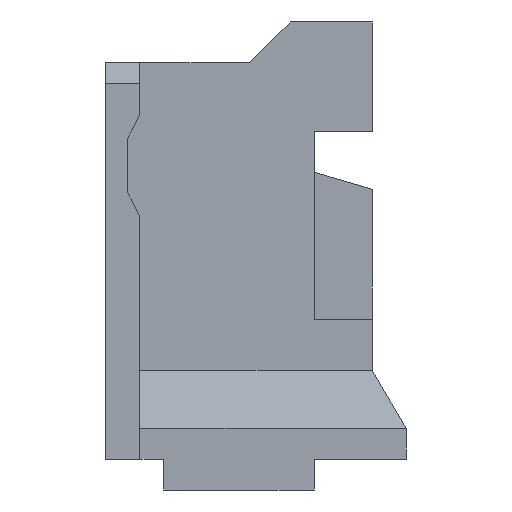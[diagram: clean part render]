
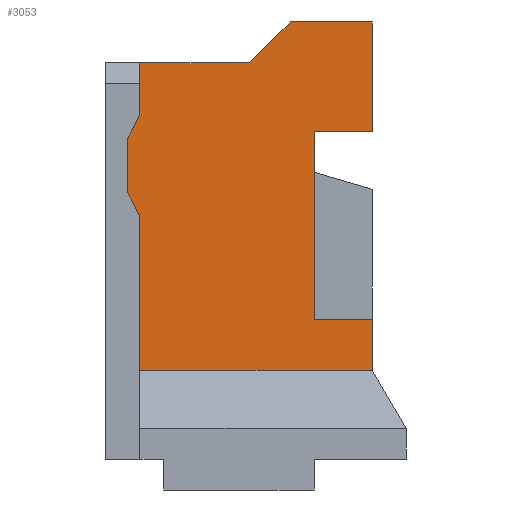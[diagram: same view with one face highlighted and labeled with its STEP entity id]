
A CAD part, left-side view. The second image highlights one B-rep face of the part: STEP entity #3053.
In plain terms, the highlighted planar face has unit normal (-1, 0, 0).
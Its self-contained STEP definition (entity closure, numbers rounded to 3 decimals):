
#169 = VERTEX_POINT ( 'NONE', #1903 ) ;
#191 = EDGE_CURVE ( 'NONE', #169, #4193, #7744, .T. ) ;
#221 = CARTESIAN_POINT ( 'NONE',  ( -1.25, 1.275, -1.9 ) ) ;
#229 = CARTESIAN_POINT ( 'NONE',  ( -1.25, -2.3, -1. ) ) ;
#262 = DIRECTION ( 'NONE',  ( 0., 0., -1. ) ) ;
#486 = EDGE_CURVE ( 'NONE', #6037, #6404, #1408, .T. ) ;
#493 = ORIENTED_EDGE ( 'NONE', *, *, #486, .F. ) ;
#545 = AXIS2_PLACEMENT_3D ( 'NONE', #3098, #8033, #262 ) ;
#607 = VECTOR ( 'NONE', #777, 1000. ) ;
#658 = FACE_OUTER_BOUND ( 'NONE', #4028, .T. ) ;
#683 = CARTESIAN_POINT ( 'NONE',  ( -1.25, -0.5, 0. ) ) ;
#768 = VECTOR ( 'NONE', #8180, 1000. ) ;
#777 = DIRECTION ( 'NONE',  ( 0., 0., -1. ) ) ;
#843 = LINE ( 'NONE', #988, #3756 ) ;
#858 = CARTESIAN_POINT ( 'NONE',  ( -1.25, -2.3, 0.6 ) ) ;
#988 = CARTESIAN_POINT ( 'NONE',  ( -1.25, 1.275, -2.25 ) ) ;
#1013 = VERTEX_POINT ( 'NONE', #683 ) ;
#1049 = LINE ( 'NONE', #7184, #607 ) ;
#1170 = VECTOR ( 'NONE', #2910, 1000. ) ;
#1318 = EDGE_CURVE ( 'NONE', #1013, #2790, #4497, .T. ) ;
#1408 = LINE ( 'NONE', #4953, #3668 ) ;
#1420 = ORIENTED_EDGE ( 'NONE', *, *, #191, .F. ) ;
#1621 = LINE ( 'NONE', #4563, #2403 ) ;
#1644 = EDGE_CURVE ( 'NONE', #5227, #169, #7992, .T. ) ;
#1797 = DIRECTION ( 'NONE',  ( 0., 0., 1. ) ) ;
#1844 = ORIENTED_EDGE ( 'NONE', *, *, #3204, .F. ) ;
#1848 = DIRECTION ( 'NONE',  ( 0., -0.707, 0.707 ) ) ;
#1903 = CARTESIAN_POINT ( 'NONE',  ( -1.25, -2.3, -4.5 ) ) ;
#1930 = CARTESIAN_POINT ( 'NONE',  ( -1.25, 1.1, -4.5 ) ) ;
#2403 = VECTOR ( 'NONE', #1797, 1000. ) ;
#2417 = VECTOR ( 'NONE', #2526, 1000. ) ;
#2526 = DIRECTION ( 'NONE',  ( 0., 1., 0. ) ) ;
#2658 = LINE ( 'NONE', #3257, #768 ) ;
#2671 = EDGE_CURVE ( 'NONE', #2914, #4489, #6462, .T. ) ;
#2777 = VECTOR ( 'NONE', #8458, 1000. ) ;
#2790 = VERTEX_POINT ( 'NONE', #4265 ) ;
#2888 = CARTESIAN_POINT ( 'NONE',  ( -1.25, 1.1, -2.25 ) ) ;
#2910 = DIRECTION ( 'NONE',  ( 0., -1., 0. ) ) ;
#2914 = VERTEX_POINT ( 'NONE', #2888 ) ;
#3053 = ADVANCED_FACE ( 'NONE', ( #658 ), #4514, .F. ) ;
#3098 = CARTESIAN_POINT ( 'NONE',  ( -1.25, 0., 0. ) ) ;
#3102 = VECTOR ( 'NONE', #6537, 1000. ) ;
#3204 = EDGE_CURVE ( 'NONE', #6404, #5682, #8960, .T. ) ;
#3217 = EDGE_CURVE ( 'NONE', #8971, #5227, #2658, .T. ) ;
#3257 = CARTESIAN_POINT ( 'NONE',  ( -1.25, 3.057, -3.75 ) ) ;
#3654 = LINE ( 'NONE', #858, #9047 ) ;
#3658 = VERTEX_POINT ( 'NONE', #4592 ) ;
#3668 = VECTOR ( 'NONE', #7849, 1000. ) ;
#3673 = ORIENTED_EDGE ( 'NONE', *, *, #4597, .F. ) ;
#3756 = VECTOR ( 'NONE', #8781, 1000. ) ;
#3965 = CARTESIAN_POINT ( 'NONE',  ( -1.25, 1.1, -5.8 ) ) ;
#4020 = EDGE_CURVE ( 'NONE', #2790, #3658, #5007, .T. ) ;
#4028 = EDGE_LOOP ( 'NONE', ( #1844, #493, #7671, #8993, #3673, #1420, #7747, #4787, #8185, #7156, #5401, #6274, #6534, #6407 ) ) ;
#4114 = EDGE_CURVE ( 'NONE', #4242, #5661, #8613, .T. ) ;
#4145 = VECTOR ( 'NONE', #1848, 1000. ) ;
#4193 = VERTEX_POINT ( 'NONE', #1930 ) ;
#4242 = VERTEX_POINT ( 'NONE', #6969 ) ;
#4265 = CARTESIAN_POINT ( 'NONE',  ( -1.25, -1.1, 0.6 ) ) ;
#4307 = DIRECTION ( 'NONE',  ( 0., 0., -1. ) ) ;
#4348 = EDGE_CURVE ( 'NONE', #5682, #1013, #5214, .T. ) ;
#4487 = VECTOR ( 'NONE', #4307, 1000. ) ;
#4489 = VERTEX_POINT ( 'NONE', #221 ) ;
#4497 = LINE ( 'NONE', #8996, #4145 ) ;
#4514 = PLANE ( 'NONE',  #545 ) ;
#4563 = CARTESIAN_POINT ( 'NONE',  ( -1.25, 1.1, -5.8 ) ) ;
#4592 = CARTESIAN_POINT ( 'NONE',  ( -1.25, -2.3, 0.6 ) ) ;
#4597 = EDGE_CURVE ( 'NONE', #4193, #2914, #1621, .T. ) ;
#4664 = EDGE_CURVE ( 'NONE', #4489, #6037, #843, .T. ) ;
#4666 = VECTOR ( 'NONE', #5222, 1000. ) ;
#4787 = ORIENTED_EDGE ( 'NONE', *, *, #3217, .F. ) ;
#4931 = CARTESIAN_POINT ( 'NONE',  ( -1.25, 1.1, -2.25 ) ) ;
#4953 = CARTESIAN_POINT ( 'NONE',  ( -1.25, 1.1, -0.75 ) ) ;
#5007 = LINE ( 'NONE', #5887, #3102 ) ;
#5075 = CARTESIAN_POINT ( 'NONE',  ( -1.25, -1.45, -1. ) ) ;
#5214 = LINE ( 'NONE', #6350, #1170 ) ;
#5222 = DIRECTION ( 'NONE',  ( 0., 1., 0. ) ) ;
#5227 = VERTEX_POINT ( 'NONE', #6052 ) ;
#5401 = ORIENTED_EDGE ( 'NONE', *, *, #7777, .F. ) ;
#5661 = VERTEX_POINT ( 'NONE', #5075 ) ;
#5682 = VERTEX_POINT ( 'NONE', #8590 ) ;
#5778 = VECTOR ( 'NONE', #8881, 1000. ) ;
#5887 = CARTESIAN_POINT ( 'NONE',  ( -1.25, -1.1, 0.6 ) ) ;
#6037 = VERTEX_POINT ( 'NONE', #6994 ) ;
#6052 = CARTESIAN_POINT ( 'NONE',  ( -1.25, -2.3, -3.75 ) ) ;
#6274 = ORIENTED_EDGE ( 'NONE', *, *, #4020, .F. ) ;
#6350 = CARTESIAN_POINT ( 'NONE',  ( -1.25, 1.1, 0. ) ) ;
#6404 = VERTEX_POINT ( 'NONE', #8135 ) ;
#6407 = ORIENTED_EDGE ( 'NONE', *, *, #4348, .F. ) ;
#6462 = LINE ( 'NONE', #4931, #2777 ) ;
#6517 = CARTESIAN_POINT ( 'NONE',  ( -1.25, -2.3, -1.85 ) ) ;
#6534 = ORIENTED_EDGE ( 'NONE', *, *, #1318, .F. ) ;
#6537 = DIRECTION ( 'NONE',  ( 0., -1., 0. ) ) ;
#6969 = CARTESIAN_POINT ( 'NONE',  ( -1.25, -2.3, -1. ) ) ;
#6994 = CARTESIAN_POINT ( 'NONE',  ( -1.25, 1.275, -1.1 ) ) ;
#7156 = ORIENTED_EDGE ( 'NONE', *, *, #4114, .F. ) ;
#7184 = CARTESIAN_POINT ( 'NONE',  ( -1.25, -1.45, -1. ) ) ;
#7671 = ORIENTED_EDGE ( 'NONE', *, *, #4664, .F. ) ;
#7744 = LINE ( 'NONE', #8887, #2417 ) ;
#7747 = ORIENTED_EDGE ( 'NONE', *, *, #1644, .F. ) ;
#7777 = EDGE_CURVE ( 'NONE', #3658, #4242, #3654, .T. ) ;
#7849 = DIRECTION ( 'NONE',  ( 0., -0.447, 0.894 ) ) ;
#7992 = LINE ( 'NONE', #6517, #4487 ) ;
#8033 = DIRECTION ( 'NONE',  ( 1., 0., 0. ) ) ;
#8135 = CARTESIAN_POINT ( 'NONE',  ( -1.25, 1.1, -0.75 ) ) ;
#8180 = DIRECTION ( 'NONE',  ( 0., -1., 0. ) ) ;
#8185 = ORIENTED_EDGE ( 'NONE', *, *, #8532, .F. ) ;
#8458 = DIRECTION ( 'NONE',  ( 0., 0.447, 0.894 ) ) ;
#8532 = EDGE_CURVE ( 'NONE', #5661, #8971, #1049, .T. ) ;
#8577 = DIRECTION ( 'NONE',  ( 0., 0., -1. ) ) ;
#8590 = CARTESIAN_POINT ( 'NONE',  ( -1.25, 1.1, 0. ) ) ;
#8613 = LINE ( 'NONE', #229, #4666 ) ;
#8743 = CARTESIAN_POINT ( 'NONE',  ( -1.25, -1.45, -3.75 ) ) ;
#8781 = DIRECTION ( 'NONE',  ( 0., 0., 1. ) ) ;
#8881 = DIRECTION ( 'NONE',  ( 0., 0., 1. ) ) ;
#8887 = CARTESIAN_POINT ( 'NONE',  ( -1.25, -3., -4.5 ) ) ;
#8960 = LINE ( 'NONE', #3965, #5778 ) ;
#8971 = VERTEX_POINT ( 'NONE', #8743 ) ;
#8993 = ORIENTED_EDGE ( 'NONE', *, *, #2671, .F. ) ;
#8996 = CARTESIAN_POINT ( 'NONE',  ( -1.25, -0.5, 0. ) ) ;
#9047 = VECTOR ( 'NONE', #8577, 1000. ) ;
